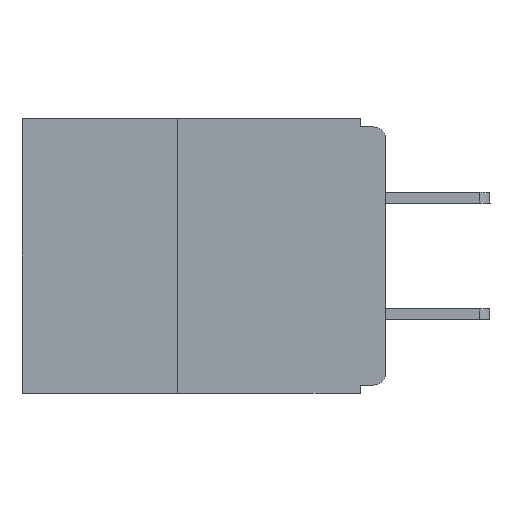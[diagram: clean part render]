
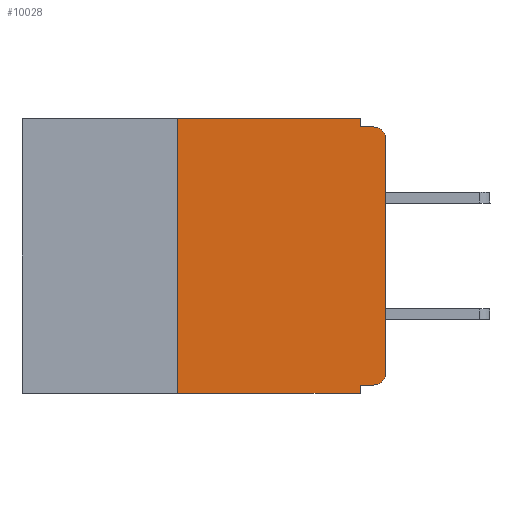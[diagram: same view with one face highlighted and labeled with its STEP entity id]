
A CAD part, left-side view. The second image highlights one B-rep face of the part: STEP entity #10028.
In plain terms, the highlighted planar face has unit normal (-1, 0, 0).
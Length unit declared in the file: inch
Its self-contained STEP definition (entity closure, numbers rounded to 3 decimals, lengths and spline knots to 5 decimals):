
#155 = CARTESIAN_POINT ( 'NONE',  ( 0., 0.015, -0.025 ) ) ;
#157 = CARTESIAN_POINT ( 'NONE',  ( 0., 0., -0.025 ) ) ;
#159 = CARTESIAN_POINT ( 'NONE',  ( 0., 0.25, -0.33 ) ) ;
#160 = DIRECTION ( 'NONE',  ( -1., 0., 0. ) ) ;
#180 = VECTOR ( 'NONE', #2900, 39.37008 ) ;
#321 = DIRECTION ( 'NONE',  ( 0., 0., -1. ) ) ;
#322 = DIRECTION ( 'NONE',  ( 0., 0., -1. ) ) ;
#358 = DIRECTION ( 'NONE',  ( 0., 0., -1. ) ) ;
#368 = EDGE_CURVE ( 'NONE', #9325, #2067, #7818, .T. ) ;
#933 = LINE ( 'NONE', #4220, #6870 ) ;
#954 = DIRECTION ( 'NONE',  ( 0., -1., 0. ) ) ;
#1105 = ORIENTED_EDGE ( 'NONE', *, *, #2825, .F. ) ;
#1228 = CARTESIAN_POINT ( 'NONE',  ( 0., 0.031, -0.33 ) ) ;
#1405 = VECTOR ( 'NONE', #10794, 39.37008 ) ;
#1487 = ORIENTED_EDGE ( 'NONE', *, *, #8937, .F. ) ;
#1657 = PLANE ( 'NONE',  #7433 ) ;
#1678 = VERTEX_POINT ( 'NONE', #9152 ) ;
#1884 = CARTESIAN_POINT ( 'NONE',  ( 0., 0.437, 0. ) ) ;
#2032 = VERTEX_POINT ( 'NONE', #6414 ) ;
#2050 = VERTEX_POINT ( 'NONE', #6611 ) ;
#2067 = VERTEX_POINT ( 'NONE', #12165 ) ;
#2184 = ORIENTED_EDGE ( 'NONE', *, *, #4096, .F. ) ;
#2425 = CARTESIAN_POINT ( 'NONE',  ( 0., 0., -0.01 ) ) ;
#2523 = LINE ( 'NONE', #159, #5723 ) ;
#2825 = EDGE_CURVE ( 'NONE', #1678, #2067, #6289, .T. ) ;
#2900 = DIRECTION ( 'NONE',  ( 0., -1., 0. ) ) ;
#3081 = VERTEX_POINT ( 'NONE', #10310 ) ;
#3109 = ORIENTED_EDGE ( 'NONE', *, *, #3360, .T. ) ;
#3360 = EDGE_CURVE ( 'NONE', #9917, #2050, #10239, .T. ) ;
#3657 = FACE_OUTER_BOUND ( 'NONE', #4813, .T. ) ;
#3718 = AXIS2_PLACEMENT_3D ( 'NONE', #5753, #160, #6668 ) ;
#3904 = LINE ( 'NONE', #2425, #7707 ) ;
#3909 = ORIENTED_EDGE ( 'NONE', *, *, #8065, .F. ) ;
#3955 = ORIENTED_EDGE ( 'NONE', *, *, #368, .T. ) ;
#4060 = CARTESIAN_POINT ( 'NONE',  ( 0., 0.031, 0. ) ) ;
#4096 = EDGE_CURVE ( 'NONE', #11309, #2050, #3904, .T. ) ;
#4192 = ORIENTED_EDGE ( 'NONE', *, *, #7950, .F. ) ;
#4220 = CARTESIAN_POINT ( 'NONE',  ( 0., 0., -0.32 ) ) ;
#4607 = CIRCLE ( 'NONE', #3718, 0.015 ) ;
#4813 = EDGE_LOOP ( 'NONE', ( #8554, #3109, #2184, #3909, #1487, #4192, #3955, #1105, #7924, #8342 ) ) ;
#4982 = LINE ( 'NONE', #4060, #7783 ) ;
#4995 = EDGE_CURVE ( 'NONE', #6296, #10350, #4607, .T. ) ;
#5119 = LINE ( 'NONE', #1884, #180 ) ;
#5473 = DIRECTION ( 'NONE',  ( 1., 0., 0. ) ) ;
#5509 = EDGE_CURVE ( 'NONE', #10350, #9917, #6934, .T. ) ;
#5723 = VECTOR ( 'NONE', #11430, 39.37008 ) ;
#5753 = CARTESIAN_POINT ( 'NONE',  ( 0., 0.015, -0.305 ) ) ;
#5938 = CARTESIAN_POINT ( 'NONE',  ( 0., 0., 0. ) ) ;
#6049 = DIRECTION ( 'NONE',  ( 0., -1., 0. ) ) ;
#6203 = VECTOR ( 'NONE', #954, 39.37008 ) ;
#6289 = LINE ( 'NONE', #1228, #8511 ) ;
#6296 = VERTEX_POINT ( 'NONE', #9216 ) ;
#6414 = CARTESIAN_POINT ( 'NONE',  ( 0., 0.25, 0. ) ) ;
#6509 = AXIS2_PLACEMENT_3D ( 'NONE', #155, #10599, #358 ) ;
#6611 = CARTESIAN_POINT ( 'NONE',  ( 0., 0.015, -0.01 ) ) ;
#6668 = DIRECTION ( 'NONE',  ( 0., 0., -1. ) ) ;
#6870 = VECTOR ( 'NONE', #6947, 39.37008 ) ;
#6934 = LINE ( 'NONE', #5938, #1405 ) ;
#6947 = DIRECTION ( 'NONE',  ( 0., 1., 0. ) ) ;
#7255 = CARTESIAN_POINT ( 'NONE',  ( 0., 0.437, 0. ) ) ;
#7433 = AXIS2_PLACEMENT_3D ( 'NONE', #7255, #5473, #11164 ) ;
#7707 = VECTOR ( 'NONE', #6049, 39.37008 ) ;
#7783 = VECTOR ( 'NONE', #321, 39.37008 ) ;
#7818 = LINE ( 'NONE', #8464, #6203 ) ;
#7924 = ORIENTED_EDGE ( 'NONE', *, *, #8223, .F. ) ;
#7950 = EDGE_CURVE ( 'NONE', #9325, #2032, #2523, .T. ) ;
#8065 = EDGE_CURVE ( 'NONE', #3081, #11309, #4982, .T. ) ;
#8223 = EDGE_CURVE ( 'NONE', #6296, #1678, #933, .T. ) ;
#8342 = ORIENTED_EDGE ( 'NONE', *, *, #4995, .T. ) ;
#8464 = CARTESIAN_POINT ( 'NONE',  ( 0., 0.437, -0.33 ) ) ;
#8511 = VECTOR ( 'NONE', #322, 39.37008 ) ;
#8554 = ORIENTED_EDGE ( 'NONE', *, *, #5509, .T. ) ;
#8937 = EDGE_CURVE ( 'NONE', #2032, #3081, #5119, .T. ) ;
#9072 = CARTESIAN_POINT ( 'NONE',  ( 0., 0., -0.305 ) ) ;
#9152 = CARTESIAN_POINT ( 'NONE',  ( 0., 0.031, -0.32 ) ) ;
#9216 = CARTESIAN_POINT ( 'NONE',  ( 0., 0.015, -0.32 ) ) ;
#9325 = VERTEX_POINT ( 'NONE', #11608 ) ;
#9826 = CARTESIAN_POINT ( 'NONE',  ( 0., 0.031, -0.01 ) ) ;
#9917 = VERTEX_POINT ( 'NONE', #157 ) ;
#10028 = ADVANCED_FACE ( 'NONE', ( #3657 ), #1657, .F. ) ;
#10239 = CIRCLE ( 'NONE', #6509, 0.015 ) ;
#10310 = CARTESIAN_POINT ( 'NONE',  ( 0., 0.031, 0. ) ) ;
#10350 = VERTEX_POINT ( 'NONE', #9072 ) ;
#10599 = DIRECTION ( 'NONE',  ( -1., 0., 0. ) ) ;
#10794 = DIRECTION ( 'NONE',  ( 0., 0., 1. ) ) ;
#11164 = DIRECTION ( 'NONE',  ( 0., 0., -1. ) ) ;
#11309 = VERTEX_POINT ( 'NONE', #9826 ) ;
#11430 = DIRECTION ( 'NONE',  ( 0., 0., 1. ) ) ;
#11608 = CARTESIAN_POINT ( 'NONE',  ( 0., 0.25, -0.33 ) ) ;
#12165 = CARTESIAN_POINT ( 'NONE',  ( 0., 0.031, -0.33 ) ) ;
